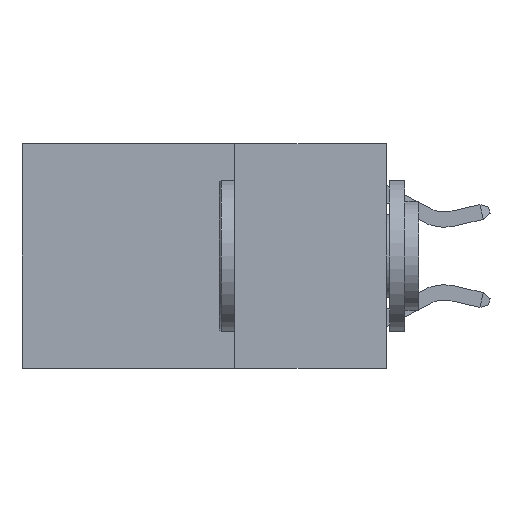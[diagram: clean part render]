
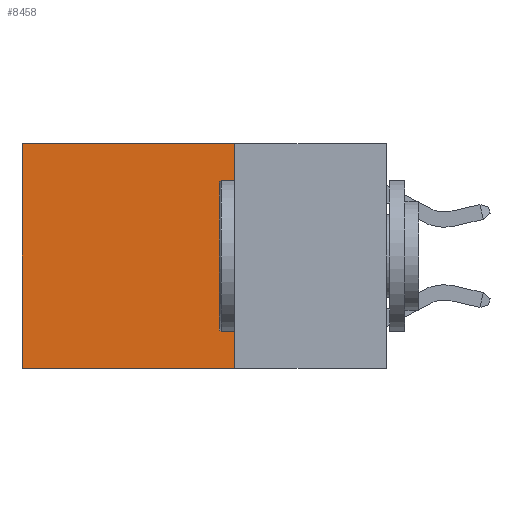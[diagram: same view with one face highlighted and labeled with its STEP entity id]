
A CAD part, left-side view. The second image highlights one B-rep face of the part: STEP entity #8458.
In plain terms, the highlighted planar face has unit normal (-1, 0, 0).
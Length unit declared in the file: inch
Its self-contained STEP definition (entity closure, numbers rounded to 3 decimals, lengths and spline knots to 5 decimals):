
#1028 = CARTESIAN_POINT ( 'NONE',  ( 0.2625, 0.25, 0. ) ) ;
#1664 = DIRECTION ( 'NONE',  ( 0., 1., 0. ) ) ;
#1995 = DIRECTION ( 'NONE',  ( 0., 0., -1. ) ) ;
#2417 = LINE ( 'NONE', #5858, #17333 ) ;
#2712 = DIRECTION ( 'NONE',  ( 1., 0., 0. ) ) ;
#2772 = EDGE_CURVE ( 'NONE', #17359, #17524, #5830, .T. ) ;
#2799 = DIRECTION ( 'NONE',  ( 0., 1., 0. ) ) ;
#3196 = CARTESIAN_POINT ( 'NONE',  ( 0.2625, 0.25, 0. ) ) ;
#4052 = DIRECTION ( 'NONE',  ( 0., 0., -1. ) ) ;
#4213 = CARTESIAN_POINT ( 'NONE',  ( 0.2625, 0.25, 0. ) ) ;
#4342 = ORIENTED_EDGE ( 'NONE', *, *, #4462, .T. ) ;
#4462 = EDGE_CURVE ( 'NONE', #11112, #15318, #12358, .T. ) ;
#5830 = LINE ( 'NONE', #11579, #10690 ) ;
#5858 = CARTESIAN_POINT ( 'NONE',  ( 0.2625, 0.6, 0. ) ) ;
#5878 = CARTESIAN_POINT ( 'NONE',  ( 0.2625, 0.25, 0. ) ) ;
#7851 = ORIENTED_EDGE ( 'NONE', *, *, #15682, .T. ) ;
#8458 = ADVANCED_FACE ( 'NONE', ( #13395 ), #18026, .F. ) ;
#8696 = LINE ( 'NONE', #5878, #14737 ) ;
#9870 = EDGE_CURVE ( 'NONE', #11112, #17359, #8696, .T. ) ;
#10690 = VECTOR ( 'NONE', #2799, 39.37008 ) ;
#11112 = VERTEX_POINT ( 'NONE', #1028 ) ;
#11276 = EDGE_LOOP ( 'NONE', ( #7851, #14898, #16828, #4342 ) ) ;
#11579 = CARTESIAN_POINT ( 'NONE',  ( 0.2625, 0.25, -0.37 ) ) ;
#12358 = LINE ( 'NONE', #3196, #14273 ) ;
#13395 = FACE_OUTER_BOUND ( 'NONE', #11276, .T. ) ;
#13664 = CARTESIAN_POINT ( 'NONE',  ( 0.2625, 0.6, -0.37 ) ) ;
#14273 = VECTOR ( 'NONE', #1664, 39.37008 ) ;
#14737 = VECTOR ( 'NONE', #19600, 39.37008 ) ;
#14898 = ORIENTED_EDGE ( 'NONE', *, *, #2772, .F. ) ;
#15318 = VERTEX_POINT ( 'NONE', #17158 ) ;
#15682 = EDGE_CURVE ( 'NONE', #15318, #17524, #2417, .T. ) ;
#15892 = AXIS2_PLACEMENT_3D ( 'NONE', #4213, #2712, #1995 ) ;
#16828 = ORIENTED_EDGE ( 'NONE', *, *, #9870, .F. ) ;
#17158 = CARTESIAN_POINT ( 'NONE',  ( 0.2625, 0.6, 0. ) ) ;
#17333 = VECTOR ( 'NONE', #4052, 39.37008 ) ;
#17359 = VERTEX_POINT ( 'NONE', #17698 ) ;
#17524 = VERTEX_POINT ( 'NONE', #13664 ) ;
#17698 = CARTESIAN_POINT ( 'NONE',  ( 0.2625, 0.25, -0.37 ) ) ;
#18026 = PLANE ( 'NONE',  #15892 ) ;
#19600 = DIRECTION ( 'NONE',  ( 0., 0., -1. ) ) ;
